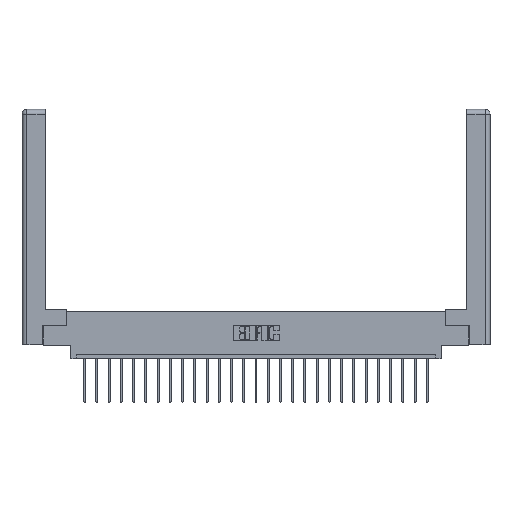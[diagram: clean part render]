
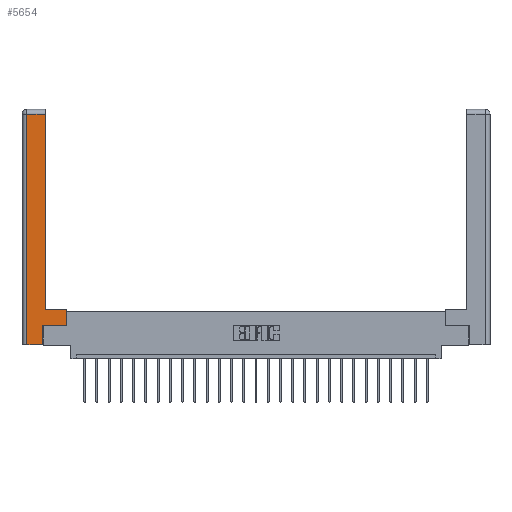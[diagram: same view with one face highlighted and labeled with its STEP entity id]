
A CAD part, top view. The second image highlights one B-rep face of the part: STEP entity #5654.
In plain terms, the highlighted planar face has unit normal (0, 0, 1).
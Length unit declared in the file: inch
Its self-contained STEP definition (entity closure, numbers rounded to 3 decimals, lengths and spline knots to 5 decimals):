
#157 = DIRECTION ( 'NONE',  ( 0., 1., 0. ) ) ;
#1392 = LINE ( 'NONE', #25692, #20550 ) ;
#1865 = VERTEX_POINT ( 'NONE', #19478 ) ;
#2085 = ORIENTED_EDGE ( 'NONE', *, *, #8703, .T. ) ;
#2326 = AXIS2_PLACEMENT_3D ( 'NONE', #6693, #8705, #24531 ) ;
#2368 = VECTOR ( 'NONE', #5062, 39.37008 ) ;
#3202 = VECTOR ( 'NONE', #20794, 39.37008 ) ;
#3666 = DIRECTION ( 'NONE',  ( -1., 0., 0. ) ) ;
#3902 = VERTEX_POINT ( 'NONE', #20451 ) ;
#4377 = EDGE_LOOP ( 'NONE', ( #15438, #7672, #10136, #2085, #25289, #8384, #16297, #18180 ) ) ;
#4682 = EDGE_CURVE ( 'NONE', #14252, #23058, #15281, .T. ) ;
#4775 = DIRECTION ( 'NONE',  ( 0., 1., 0. ) ) ;
#4778 = FACE_OUTER_BOUND ( 'NONE', #4377, .T. ) ;
#4854 = CARTESIAN_POINT ( 'NONE',  ( 0.265, 0.245, 0. ) ) ;
#4939 = LINE ( 'NONE', #15145, #23170 ) ;
#5062 = DIRECTION ( 'NONE',  ( 1., 0., 0. ) ) ;
#5654 = ADVANCED_FACE ( 'NONE', ( #4778 ), #12768, .F. ) ;
#5825 = CARTESIAN_POINT ( 'NONE',  ( 0.295, 0.45, 0. ) ) ;
#6014 = VERTEX_POINT ( 'NONE', #8081 ) ;
#6391 = CARTESIAN_POINT ( 'NONE',  ( 0.565, 0.245, 0. ) ) ;
#6693 = CARTESIAN_POINT ( 'NONE',  ( 0., 0., 0. ) ) ;
#7424 = EDGE_CURVE ( 'NONE', #6014, #20499, #11270, .T. ) ;
#7672 = ORIENTED_EDGE ( 'NONE', *, *, #10466, .T. ) ;
#7884 = CARTESIAN_POINT ( 'NONE',  ( 0.0615, 0., 0. ) ) ;
#8081 = CARTESIAN_POINT ( 'NONE',  ( 0.565, 0.45, 0. ) ) ;
#8384 = ORIENTED_EDGE ( 'NONE', *, *, #4682, .T. ) ;
#8703 = EDGE_CURVE ( 'NONE', #3902, #9362, #9636, .T. ) ;
#8705 = DIRECTION ( 'NONE',  ( 0., 0., -1. ) ) ;
#9362 = VERTEX_POINT ( 'NONE', #14356 ) ;
#9636 = LINE ( 'NONE', #23779, #11221 ) ;
#10136 = ORIENTED_EDGE ( 'NONE', *, *, #21877, .T. ) ;
#10170 = LINE ( 'NONE', #12192, #12705 ) ;
#10466 = EDGE_CURVE ( 'NONE', #1865, #25723, #1392, .T. ) ;
#10508 = EDGE_CURVE ( 'NONE', #9362, #14252, #10170, .T. ) ;
#11221 = VECTOR ( 'NONE', #19933, 39.37008 ) ;
#11270 = LINE ( 'NONE', #22061, #19453 ) ;
#11565 = VECTOR ( 'NONE', #4775, 39.37008 ) ;
#12192 = CARTESIAN_POINT ( 'NONE',  ( 0.265, 0.245, 0. ) ) ;
#12705 = VECTOR ( 'NONE', #157, 39.37008 ) ;
#12768 = PLANE ( 'NONE',  #2326 ) ;
#13448 = DIRECTION ( 'NONE',  ( 0., 1., 0. ) ) ;
#14197 = LINE ( 'NONE', #7884, #3202 ) ;
#14252 = VERTEX_POINT ( 'NONE', #4854 ) ;
#14356 = CARTESIAN_POINT ( 'NONE',  ( 0.265, 0., 0. ) ) ;
#15145 = CARTESIAN_POINT ( 'NONE',  ( 0.565, 0.45, 0. ) ) ;
#15281 = LINE ( 'NONE', #18677, #2368 ) ;
#15438 = ORIENTED_EDGE ( 'NONE', *, *, #24118, .T. ) ;
#16060 = DIRECTION ( 'NONE',  ( -1., 0., 0. ) ) ;
#16297 = ORIENTED_EDGE ( 'NONE', *, *, #24688, .T. ) ;
#18180 = ORIENTED_EDGE ( 'NONE', *, *, #7424, .T. ) ;
#18677 = CARTESIAN_POINT ( 'NONE',  ( 0.565, 0.245, 0. ) ) ;
#19453 = VECTOR ( 'NONE', #16060, 39.37008 ) ;
#19478 = CARTESIAN_POINT ( 'NONE',  ( 0.295, 2.94, 0. ) ) ;
#19933 = DIRECTION ( 'NONE',  ( 1., 0., 0. ) ) ;
#20451 = CARTESIAN_POINT ( 'NONE',  ( 0.0615, 0., 0. ) ) ;
#20499 = VERTEX_POINT ( 'NONE', #5825 ) ;
#20550 = VECTOR ( 'NONE', #3666, 39.37008 ) ;
#20794 = DIRECTION ( 'NONE',  ( 0., -1., 0. ) ) ;
#21877 = EDGE_CURVE ( 'NONE', #25723, #3902, #14197, .T. ) ;
#22061 = CARTESIAN_POINT ( 'NONE',  ( 0.295, 0.45, 0. ) ) ;
#22762 = CARTESIAN_POINT ( 'NONE',  ( 0.295, 3., 0. ) ) ;
#23058 = VERTEX_POINT ( 'NONE', #6391 ) ;
#23170 = VECTOR ( 'NONE', #13448, 39.37008 ) ;
#23779 = CARTESIAN_POINT ( 'NONE',  ( 0.265, 0., 0. ) ) ;
#24118 = EDGE_CURVE ( 'NONE', #20499, #1865, #24132, .T. ) ;
#24132 = LINE ( 'NONE', #22762, #11565 ) ;
#24531 = DIRECTION ( 'NONE',  ( -1., 0., 0. ) ) ;
#24688 = EDGE_CURVE ( 'NONE', #23058, #6014, #4939, .T. ) ;
#24877 = CARTESIAN_POINT ( 'NONE',  ( 0.0615, 2.94, 0. ) ) ;
#25289 = ORIENTED_EDGE ( 'NONE', *, *, #10508, .T. ) ;
#25692 = CARTESIAN_POINT ( 'NONE',  ( 0.0615, 2.94, 0. ) ) ;
#25723 = VERTEX_POINT ( 'NONE', #24877 ) ;
